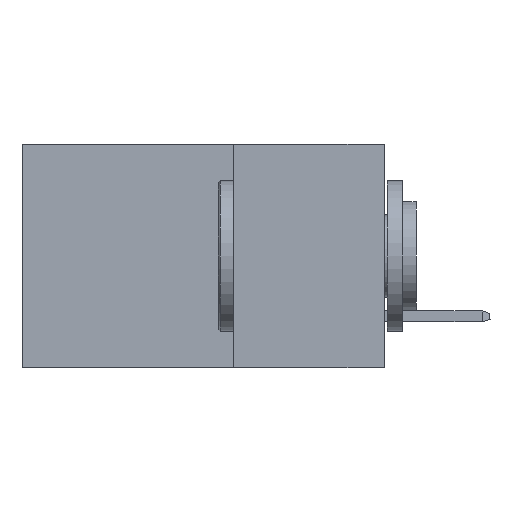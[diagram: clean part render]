
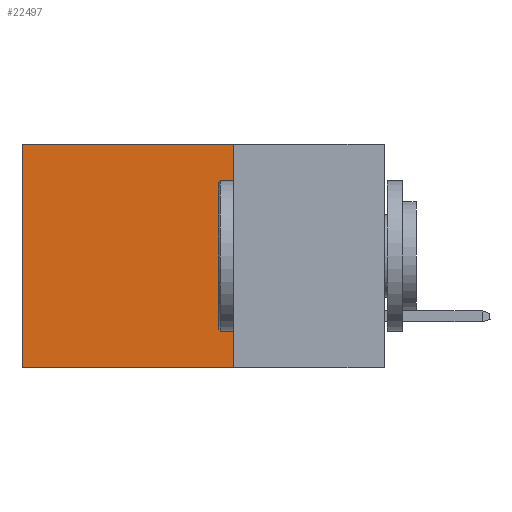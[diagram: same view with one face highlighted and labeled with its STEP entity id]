
A CAD part, left-side view. The second image highlights one B-rep face of the part: STEP entity #22497.
In plain terms, the highlighted planar face has unit normal (-1, 0, 0).
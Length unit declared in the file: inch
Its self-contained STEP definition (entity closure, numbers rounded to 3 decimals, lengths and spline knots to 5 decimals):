
#56 = FACE_OUTER_BOUND ( 'NONE', #16614, .T. ) ;
#620 = CARTESIAN_POINT ( 'NONE',  ( 0.298, 0.6, -0.37 ) ) ;
#626 = ORIENTED_EDGE ( 'NONE', *, *, #3112, .F. ) ;
#1470 = CARTESIAN_POINT ( 'NONE',  ( 0.298, 0.25, 0. ) ) ;
#3050 = EDGE_CURVE ( 'NONE', #4264, #9306, #25084, .T. ) ;
#3112 = EDGE_CURVE ( 'NONE', #4461, #9795, #5732, .T. ) ;
#3274 = PLANE ( 'NONE',  #18265 ) ;
#3565 = CARTESIAN_POINT ( 'NONE',  ( 0.298, 0.25, -0.37 ) ) ;
#4264 = VERTEX_POINT ( 'NONE', #16861 ) ;
#4461 = VERTEX_POINT ( 'NONE', #7782 ) ;
#5732 = LINE ( 'NONE', #1470, #9339 ) ;
#5921 = CARTESIAN_POINT ( 'NONE',  ( 0.298, 0.6, 0. ) ) ;
#5941 = DIRECTION ( 'NONE',  ( 0., 1., 0. ) ) ;
#7782 = CARTESIAN_POINT ( 'NONE',  ( 0.298, 0.25, 0. ) ) ;
#8161 = DIRECTION ( 'NONE',  ( 0., 1., 0. ) ) ;
#9006 = VECTOR ( 'NONE', #8161, 39.37008 ) ;
#9127 = ORIENTED_EDGE ( 'NONE', *, *, #12066, .T. ) ;
#9306 = VERTEX_POINT ( 'NONE', #620 ) ;
#9328 = LINE ( 'NONE', #18860, #13668 ) ;
#9339 = VECTOR ( 'NONE', #16320, 39.37008 ) ;
#9795 = VERTEX_POINT ( 'NONE', #25277 ) ;
#11975 = DIRECTION ( 'NONE',  ( 0., 0., -1. ) ) ;
#12066 = EDGE_CURVE ( 'NONE', #4461, #4264, #9328, .T. ) ;
#12669 = ORIENTED_EDGE ( 'NONE', *, *, #16145, .F. ) ;
#13668 = VECTOR ( 'NONE', #5941, 39.37008 ) ;
#14221 = CARTESIAN_POINT ( 'NONE',  ( 0.298, 0.25, 0. ) ) ;
#15786 = ORIENTED_EDGE ( 'NONE', *, *, #3050, .T. ) ;
#16145 = EDGE_CURVE ( 'NONE', #9795, #9306, #25414, .T. ) ;
#16320 = DIRECTION ( 'NONE',  ( 0., 0., -1. ) ) ;
#16614 = EDGE_LOOP ( 'NONE', ( #15786, #12669, #626, #9127 ) ) ;
#16861 = CARTESIAN_POINT ( 'NONE',  ( 0.298, 0.6, 0. ) ) ;
#18219 = DIRECTION ( 'NONE',  ( 1., 0., 0. ) ) ;
#18265 = AXIS2_PLACEMENT_3D ( 'NONE', #14221, #18219, #11975 ) ;
#18860 = CARTESIAN_POINT ( 'NONE',  ( 0.298, 0.25, 0. ) ) ;
#22497 = ADVANCED_FACE ( 'NONE', ( #56 ), #3274, .F. ) ;
#22729 = VECTOR ( 'NONE', #27151, 39.37008 ) ;
#25084 = LINE ( 'NONE', #5921, #22729 ) ;
#25277 = CARTESIAN_POINT ( 'NONE',  ( 0.298, 0.25, -0.37 ) ) ;
#25414 = LINE ( 'NONE', #3565, #9006 ) ;
#27151 = DIRECTION ( 'NONE',  ( 0., 0., -1. ) ) ;
